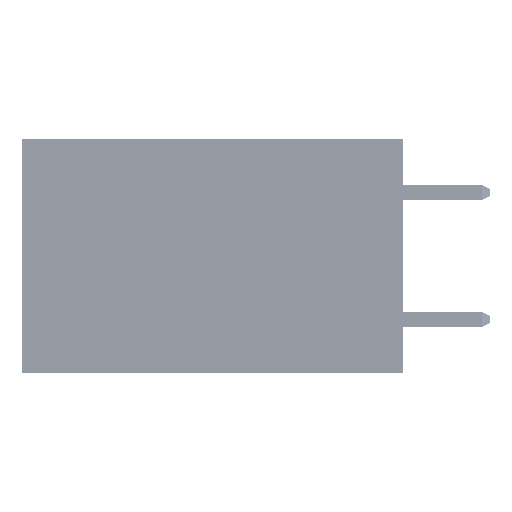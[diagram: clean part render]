
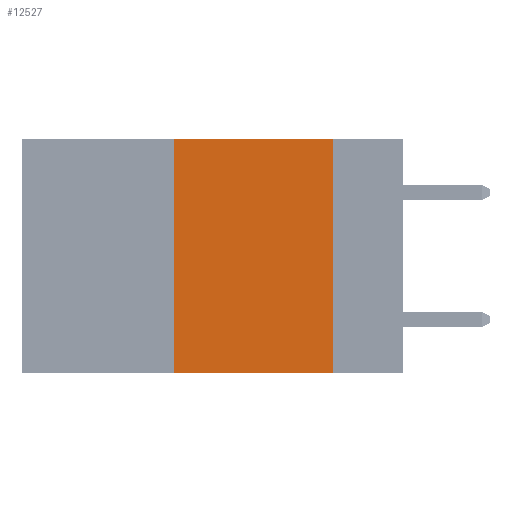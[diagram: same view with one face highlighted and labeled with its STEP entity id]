
A CAD part, left-side view. The second image highlights one B-rep face of the part: STEP entity #12527.
In plain terms, the highlighted planar face has unit normal (-1, 0, 0).
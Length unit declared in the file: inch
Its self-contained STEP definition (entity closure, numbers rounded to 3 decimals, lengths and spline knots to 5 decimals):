
#1275 = VERTEX_POINT ( 'NONE', #44944 ) ;
#3448 = EDGE_CURVE ( 'NONE', #16485, #29683, #34271, .T. ) ;
#3518 = DIRECTION ( 'NONE',  ( 0., -1., 0. ) ) ;
#4665 = DIRECTION ( 'NONE',  ( 0., -1., 0. ) ) ;
#5501 = DIRECTION ( 'NONE',  ( 0., 0., -1. ) ) ;
#5705 = CARTESIAN_POINT ( 'NONE',  ( 0., 0.6, 0. ) ) ;
#5808 = VECTOR ( 'NONE', #24275, 39.37008 ) ;
#6298 = ORIENTED_EDGE ( 'NONE', *, *, #14725, .F. ) ;
#8130 = AXIS2_PLACEMENT_3D ( 'NONE', #5705, #31945, #21012 ) ;
#8662 = CARTESIAN_POINT ( 'NONE',  ( 0., 0.36, 0. ) ) ;
#9234 = VECTOR ( 'NONE', #5501, 39.37008 ) ;
#10170 = VECTOR ( 'NONE', #3518, 39.37008 ) ;
#10478 = EDGE_CURVE ( 'NONE', #16485, #40768, #15908, .T. ) ;
#12527 = ADVANCED_FACE ( 'NONE', ( #41274 ), #24646, .F. ) ;
#12660 = CARTESIAN_POINT ( 'NONE',  ( 0., 0.36, 0. ) ) ;
#14378 = EDGE_LOOP ( 'NONE', ( #18337, #6298, #38715, #19321 ) ) ;
#14725 = EDGE_CURVE ( 'NONE', #40768, #1275, #23897, .T. ) ;
#15908 = LINE ( 'NONE', #8662, #5808 ) ;
#16485 = VERTEX_POINT ( 'NONE', #17700 ) ;
#17700 = CARTESIAN_POINT ( 'NONE',  ( 0., 0.36, -0.37 ) ) ;
#18337 = ORIENTED_EDGE ( 'NONE', *, *, #31376, .F. ) ;
#19321 = ORIENTED_EDGE ( 'NONE', *, *, #3448, .T. ) ;
#21012 = DIRECTION ( 'NONE',  ( 0., 0., -1. ) ) ;
#23620 = CARTESIAN_POINT ( 'NONE',  ( 0., 0.6, -0.37 ) ) ;
#23897 = LINE ( 'NONE', #40913, #10170 ) ;
#24275 = DIRECTION ( 'NONE',  ( 0., 0., 1. ) ) ;
#24646 = PLANE ( 'NONE',  #8130 ) ;
#27693 = LINE ( 'NONE', #28086, #9234 ) ;
#28086 = CARTESIAN_POINT ( 'NONE',  ( 0., 0.11, 0. ) ) ;
#29683 = VERTEX_POINT ( 'NONE', #40043 ) ;
#30100 = VECTOR ( 'NONE', #4665, 39.37008 ) ;
#31376 = EDGE_CURVE ( 'NONE', #1275, #29683, #27693, .T. ) ;
#31945 = DIRECTION ( 'NONE',  ( 1., 0., 0. ) ) ;
#34271 = LINE ( 'NONE', #23620, #30100 ) ;
#38715 = ORIENTED_EDGE ( 'NONE', *, *, #10478, .F. ) ;
#40043 = CARTESIAN_POINT ( 'NONE',  ( 0., 0.11, -0.37 ) ) ;
#40768 = VERTEX_POINT ( 'NONE', #12660 ) ;
#40913 = CARTESIAN_POINT ( 'NONE',  ( 0., 0.6, 0. ) ) ;
#41274 = FACE_OUTER_BOUND ( 'NONE', #14378, .T. ) ;
#44944 = CARTESIAN_POINT ( 'NONE',  ( 0., 0.11, 0. ) ) ;
